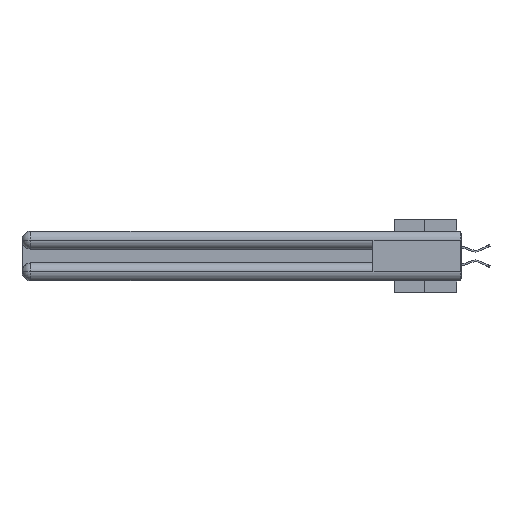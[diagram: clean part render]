
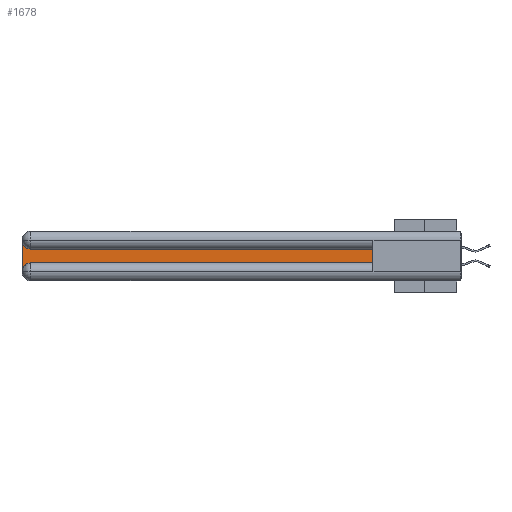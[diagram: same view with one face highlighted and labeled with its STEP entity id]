
A CAD part, left-side view. The second image highlights one B-rep face of the part: STEP entity #1678.
In plain terms, the highlighted planar face has unit normal (-1, 0, 0).
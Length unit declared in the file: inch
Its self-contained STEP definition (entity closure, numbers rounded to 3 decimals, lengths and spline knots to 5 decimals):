
#124 = CARTESIAN_POINT ( 'NONE',  ( 0.075, 3., -0.2775 ) ) ;
#893 = CARTESIAN_POINT ( 'NONE',  ( 0.075, 0.6, -0.1225 ) ) ;
#1268 = VERTEX_POINT ( 'NONE', #124 ) ;
#1678 = ADVANCED_FACE ( 'NONE', ( #14015 ), #22376, .F. ) ;
#1713 = DIRECTION ( 'NONE',  ( 0., 0., -1. ) ) ;
#2353 = DIRECTION ( 'NONE',  ( 0., 0., -1. ) ) ;
#3445 = VECTOR ( 'NONE', #13373, 39.37008 ) ;
#4413 = ORIENTED_EDGE ( 'NONE', *, *, #30363, .T. ) ;
#5119 = DIRECTION ( 'NONE',  ( 1., 0., 0. ) ) ;
#6325 = VERTEX_POINT ( 'NONE', #33346 ) ;
#6681 = DIRECTION ( 'NONE',  ( 0., 0., 1. ) ) ;
#6822 = CARTESIAN_POINT ( 'NONE',  ( 0.075, 0.6, -0.2175 ) ) ;
#6938 = EDGE_CURVE ( 'NONE', #16061, #6325, #25883, .T. ) ;
#7852 = EDGE_CURVE ( 'NONE', #23648, #25466, #23153, .T. ) ;
#8326 = CARTESIAN_POINT ( 'NONE',  ( 0.075, 2.94, -0.2775 ) ) ;
#9665 = ORIENTED_EDGE ( 'NONE', *, *, #6938, .T. ) ;
#9880 = CARTESIAN_POINT ( 'NONE',  ( 0.075, 0.6, -0.2175 ) ) ;
#9971 = VECTOR ( 'NONE', #6681, 39.37008 ) ;
#11843 = DIRECTION ( 'NONE',  ( 1., 0., 0. ) ) ;
#12763 = DIRECTION ( 'NONE',  ( 1., 0., 0. ) ) ;
#13373 = DIRECTION ( 'NONE',  ( 0., -1., 0. ) ) ;
#14015 = FACE_OUTER_BOUND ( 'NONE', #20081, .T. ) ;
#14896 = CARTESIAN_POINT ( 'NONE',  ( 0.075, 0.6, -0.1225 ) ) ;
#14914 = VECTOR ( 'NONE', #36418, 39.37008 ) ;
#15986 = CARTESIAN_POINT ( 'NONE',  ( 0.075, 3., -0.1225 ) ) ;
#16061 = VERTEX_POINT ( 'NONE', #18722 ) ;
#17173 = CARTESIAN_POINT ( 'NONE',  ( 0.075, 2.94, -0.2175 ) ) ;
#17674 = DIRECTION ( 'NONE',  ( 0., 1., 0. ) ) ;
#18722 = CARTESIAN_POINT ( 'NONE',  ( 0.075, 2.94, -0.1225 ) ) ;
#20081 = EDGE_LOOP ( 'NONE', ( #41024, #9665, #4413, #25590, #23646, #42992 ) ) ;
#21871 = DIRECTION ( 'NONE',  ( 0., 0., -1. ) ) ;
#22376 = PLANE ( 'NONE',  #24564 ) ;
#22858 = LINE ( 'NONE', #43324, #14914 ) ;
#23153 = LINE ( 'NONE', #6822, #9971 ) ;
#23646 = ORIENTED_EDGE ( 'NONE', *, *, #33742, .T. ) ;
#23648 = VERTEX_POINT ( 'NONE', #34148 ) ;
#23678 = VECTOR ( 'NONE', #17674, 39.37008 ) ;
#24564 = AXIS2_PLACEMENT_3D ( 'NONE', #15986, #12763, #2353 ) ;
#25466 = VERTEX_POINT ( 'NONE', #14896 ) ;
#25590 = ORIENTED_EDGE ( 'NONE', *, *, #34593, .T. ) ;
#25883 = CIRCLE ( 'NONE', #27819, 0.06 ) ;
#26575 = EDGE_CURVE ( 'NONE', #25466, #16061, #38339, .T. ) ;
#26760 = AXIS2_PLACEMENT_3D ( 'NONE', #8326, #11843, #21871 ) ;
#27819 = AXIS2_PLACEMENT_3D ( 'NONE', #31764, #5119, #1713 ) ;
#30363 = EDGE_CURVE ( 'NONE', #6325, #1268, #22858, .T. ) ;
#31764 = CARTESIAN_POINT ( 'NONE',  ( 0.075, 2.94, -0.0625 ) ) ;
#33346 = CARTESIAN_POINT ( 'NONE',  ( 0.075, 3., -0.0625 ) ) ;
#33742 = EDGE_CURVE ( 'NONE', #42247, #23648, #38098, .T. ) ;
#34148 = CARTESIAN_POINT ( 'NONE',  ( 0.075, 0.6, -0.2175 ) ) ;
#34593 = EDGE_CURVE ( 'NONE', #1268, #42247, #36994, .T. ) ;
#36418 = DIRECTION ( 'NONE',  ( 0., 0., -1. ) ) ;
#36994 = CIRCLE ( 'NONE', #26760, 0.06 ) ;
#38098 = LINE ( 'NONE', #9880, #3445 ) ;
#38339 = LINE ( 'NONE', #893, #23678 ) ;
#41024 = ORIENTED_EDGE ( 'NONE', *, *, #26575, .T. ) ;
#42247 = VERTEX_POINT ( 'NONE', #17173 ) ;
#42992 = ORIENTED_EDGE ( 'NONE', *, *, #7852, .T. ) ;
#43324 = CARTESIAN_POINT ( 'NONE',  ( 0.075, 3., -0.2175 ) ) ;
